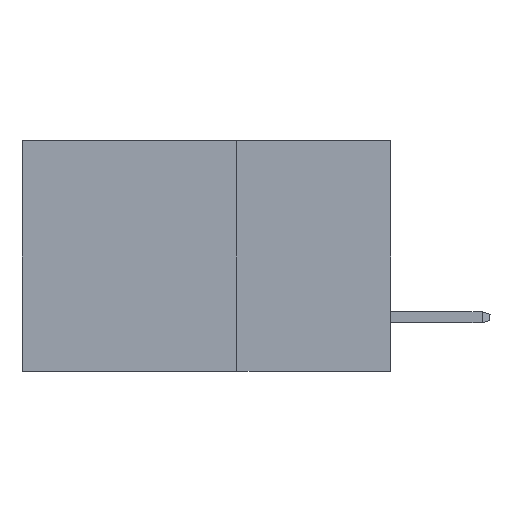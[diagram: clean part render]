
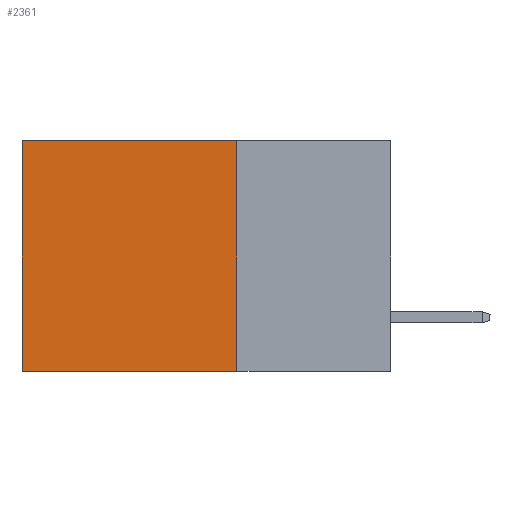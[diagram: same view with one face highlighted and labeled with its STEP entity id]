
A CAD part, left-side view. The second image highlights one B-rep face of the part: STEP entity #2361.
In plain terms, the highlighted planar face has unit normal (-1, 0, 0).
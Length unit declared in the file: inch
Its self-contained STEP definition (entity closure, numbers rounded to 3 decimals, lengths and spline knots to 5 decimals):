
#74 = VECTOR ( 'NONE', #2133, 39.37008 ) ;
#339 = DIRECTION ( 'NONE',  ( 0., 0., -1. ) ) ;
#631 = FACE_OUTER_BOUND ( 'NONE', #13725, .T. ) ;
#1496 = EDGE_CURVE ( 'NONE', #13086, #10473, #12467, .T. ) ;
#1793 = CARTESIAN_POINT ( 'NONE',  ( 0.2875, 0.25, -0.375 ) ) ;
#2090 = EDGE_CURVE ( 'NONE', #7198, #10473, #5098, .T. ) ;
#2133 = DIRECTION ( 'NONE',  ( 0., 1., 0. ) ) ;
#2361 = ADVANCED_FACE ( 'NONE', ( #631 ), #11791, .F. ) ;
#2476 = LINE ( 'NONE', #4729, #6846 ) ;
#3391 = VECTOR ( 'NONE', #7876, 39.37008 ) ;
#4215 = ORIENTED_EDGE ( 'NONE', *, *, #12946, .F. ) ;
#4381 = AXIS2_PLACEMENT_3D ( 'NONE', #1793, #10345, #339 ) ;
#4729 = CARTESIAN_POINT ( 'NONE',  ( 0.2875, 0.25, -0.375 ) ) ;
#4799 = VERTEX_POINT ( 'NONE', #5618 ) ;
#5098 = LINE ( 'NONE', #12900, #11576 ) ;
#5618 = CARTESIAN_POINT ( 'NONE',  ( 0.2875, 0.25, 0. ) ) ;
#5989 = DIRECTION ( 'NONE',  ( 0., 0., -1. ) ) ;
#6568 = ORIENTED_EDGE ( 'NONE', *, *, #1496, .F. ) ;
#6846 = VECTOR ( 'NONE', #5989, 39.37008 ) ;
#7198 = VERTEX_POINT ( 'NONE', #8860 ) ;
#7373 = DIRECTION ( 'NONE',  ( 0., 0., -1. ) ) ;
#7876 = DIRECTION ( 'NONE',  ( 0., 1., 0. ) ) ;
#8860 = CARTESIAN_POINT ( 'NONE',  ( 0.2875, 0.6, 0. ) ) ;
#10345 = DIRECTION ( 'NONE',  ( 1., 0., 0. ) ) ;
#10473 = VERTEX_POINT ( 'NONE', #12875 ) ;
#10656 = CARTESIAN_POINT ( 'NONE',  ( 0.2875, 0.25, -0.375 ) ) ;
#11025 = CARTESIAN_POINT ( 'NONE',  ( 0.2875, 0.25, 0. ) ) ;
#11172 = EDGE_CURVE ( 'NONE', #4799, #7198, #12190, .T. ) ;
#11576 = VECTOR ( 'NONE', #7373, 39.37008 ) ;
#11791 = PLANE ( 'NONE',  #4381 ) ;
#12190 = LINE ( 'NONE', #11025, #74 ) ;
#12467 = LINE ( 'NONE', #13555, #3391 ) ;
#12634 = ORIENTED_EDGE ( 'NONE', *, *, #11172, .T. ) ;
#12875 = CARTESIAN_POINT ( 'NONE',  ( 0.2875, 0.6, -0.375 ) ) ;
#12900 = CARTESIAN_POINT ( 'NONE',  ( 0.2875, 0.6, -0.375 ) ) ;
#12946 = EDGE_CURVE ( 'NONE', #4799, #13086, #2476, .T. ) ;
#13086 = VERTEX_POINT ( 'NONE', #10656 ) ;
#13518 = ORIENTED_EDGE ( 'NONE', *, *, #2090, .T. ) ;
#13555 = CARTESIAN_POINT ( 'NONE',  ( 0.2875, 0.25, -0.375 ) ) ;
#13725 = EDGE_LOOP ( 'NONE', ( #13518, #6568, #4215, #12634 ) ) ;
